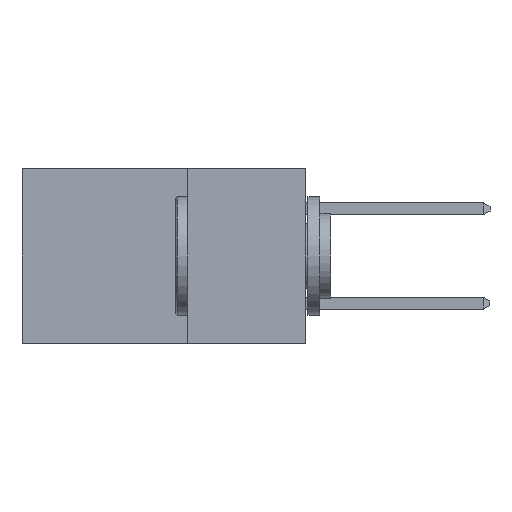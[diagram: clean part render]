
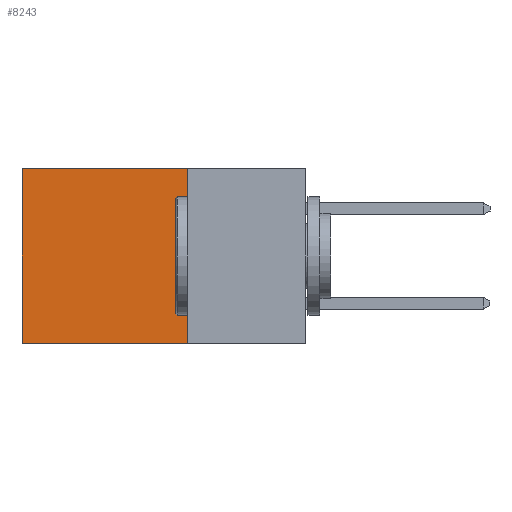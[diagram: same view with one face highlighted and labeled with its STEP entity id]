
A CAD part, left-side view. The second image highlights one B-rep face of the part: STEP entity #8243.
In plain terms, the highlighted planar face has unit normal (-1, 0, 0).
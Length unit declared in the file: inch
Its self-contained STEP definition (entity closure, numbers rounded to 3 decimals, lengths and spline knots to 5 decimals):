
#149 = ORIENTED_EDGE ( 'NONE', *, *, #12373, .T. ) ;
#473 = EDGE_LOOP ( 'NONE', ( #149, #4713, #11599, #10113 ) ) ;
#740 = LINE ( 'NONE', #8744, #10811 ) ;
#977 = VERTEX_POINT ( 'NONE', #2400 ) ;
#1116 = DIRECTION ( 'NONE',  ( 0., 0., -1. ) ) ;
#2322 = LINE ( 'NONE', #4113, #7597 ) ;
#2400 = CARTESIAN_POINT ( 'NONE',  ( 0.298, 0.6, 0. ) ) ;
#2449 = CARTESIAN_POINT ( 'NONE',  ( 0.298, 0.25, -0.37 ) ) ;
#3130 = CARTESIAN_POINT ( 'NONE',  ( 0.298, 0.25, 0. ) ) ;
#3815 = VERTEX_POINT ( 'NONE', #12378 ) ;
#4113 = CARTESIAN_POINT ( 'NONE',  ( 0.298, 0.25, 0. ) ) ;
#4127 = DIRECTION ( 'NONE',  ( 0., 0., -1. ) ) ;
#4236 = EDGE_CURVE ( 'NONE', #3815, #977, #740, .T. ) ;
#4367 = DIRECTION ( 'NONE',  ( 0., 1., 0. ) ) ;
#4703 = EDGE_CURVE ( 'NONE', #5074, #8430, #8363, .T. ) ;
#4713 = ORIENTED_EDGE ( 'NONE', *, *, #4703, .F. ) ;
#4821 = CARTESIAN_POINT ( 'NONE',  ( 0.298, 0.25, -0.37 ) ) ;
#5074 = VERTEX_POINT ( 'NONE', #2449 ) ;
#5175 = DIRECTION ( 'NONE',  ( 0., 0., -1. ) ) ;
#5312 = AXIS2_PLACEMENT_3D ( 'NONE', #3130, #9945, #4127 ) ;
#5729 = VECTOR ( 'NONE', #8316, 39.37008 ) ;
#6357 = CARTESIAN_POINT ( 'NONE',  ( 0.298, 0.6, -0.37 ) ) ;
#6769 = VECTOR ( 'NONE', #5175, 39.37008 ) ;
#7597 = VECTOR ( 'NONE', #1116, 39.37008 ) ;
#8243 = ADVANCED_FACE ( 'NONE', ( #12028 ), #9037, .F. ) ;
#8316 = DIRECTION ( 'NONE',  ( 0., 1., 0. ) ) ;
#8363 = LINE ( 'NONE', #4821, #5729 ) ;
#8430 = VERTEX_POINT ( 'NONE', #6357 ) ;
#8744 = CARTESIAN_POINT ( 'NONE',  ( 0.298, 0.25, 0. ) ) ;
#9037 = PLANE ( 'NONE',  #5312 ) ;
#9940 = LINE ( 'NONE', #9976, #6769 ) ;
#9945 = DIRECTION ( 'NONE',  ( 1., 0., 0. ) ) ;
#9976 = CARTESIAN_POINT ( 'NONE',  ( 0.298, 0.6, 0. ) ) ;
#10113 = ORIENTED_EDGE ( 'NONE', *, *, #4236, .T. ) ;
#10322 = EDGE_CURVE ( 'NONE', #3815, #5074, #2322, .T. ) ;
#10811 = VECTOR ( 'NONE', #4367, 39.37008 ) ;
#11599 = ORIENTED_EDGE ( 'NONE', *, *, #10322, .F. ) ;
#12028 = FACE_OUTER_BOUND ( 'NONE', #473, .T. ) ;
#12373 = EDGE_CURVE ( 'NONE', #977, #8430, #9940, .T. ) ;
#12378 = CARTESIAN_POINT ( 'NONE',  ( 0.298, 0.25, 0. ) ) ;
